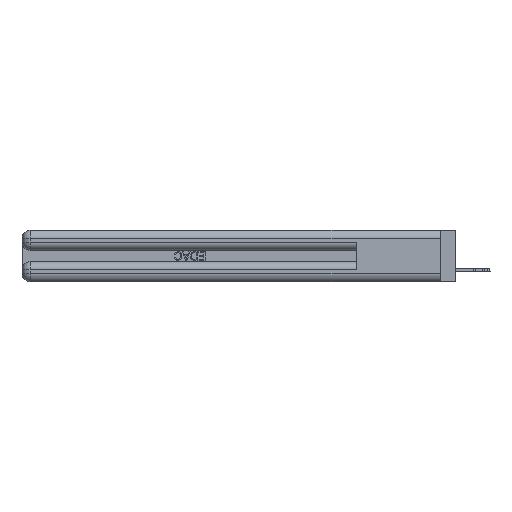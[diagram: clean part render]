
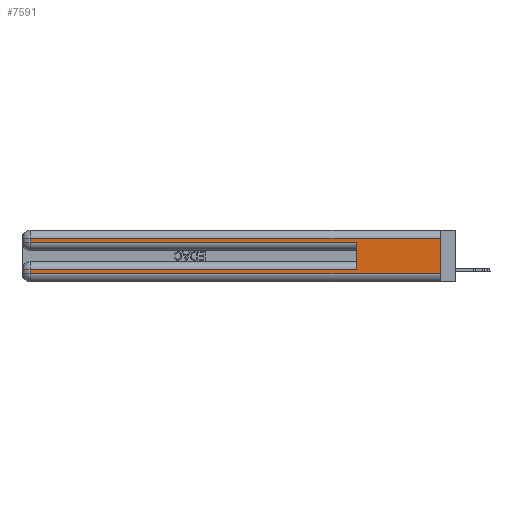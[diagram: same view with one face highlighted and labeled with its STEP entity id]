
A CAD part, left-side view. The second image highlights one B-rep face of the part: STEP entity #7591.
In plain terms, the highlighted planar face has unit normal (-1, 0, 0).
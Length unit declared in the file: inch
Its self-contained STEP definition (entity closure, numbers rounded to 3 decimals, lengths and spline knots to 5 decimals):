
#1581 = VECTOR ( 'NONE', #41209, 39.37008 ) ;
#2367 = LINE ( 'NONE', #12091, #41838 ) ;
#2590 = DIRECTION ( 'NONE',  ( 0., 0., 1. ) ) ;
#2711 = DIRECTION ( 'NONE',  ( 0., 0., -1. ) ) ;
#3112 = CARTESIAN_POINT ( 'NONE',  ( 0., 2.94, 0.06 ) ) ;
#5123 = EDGE_CURVE ( 'NONE', #44165, #44520, #13853, .T. ) ;
#5476 = VECTOR ( 'NONE', #2590, 39.37008 ) ;
#5653 = CARTESIAN_POINT ( 'NONE',  ( 0., 2.94, 0.285 ) ) ;
#5681 = LINE ( 'NONE', #5818, #33248 ) ;
#5818 = CARTESIAN_POINT ( 'NONE',  ( 0., 2.94, 0.37 ) ) ;
#6056 = CARTESIAN_POINT ( 'NONE',  ( 0., 2.94, 0.085 ) ) ;
#6322 = CARTESIAN_POINT ( 'NONE',  ( 0., 0., 0.085 ) ) ;
#6497 = EDGE_CURVE ( 'NONE', #46476, #43910, #26676, .T. ) ;
#6765 = DIRECTION ( 'NONE',  ( 1., 0., 0. ) ) ;
#7591 = ADVANCED_FACE ( 'NONE', ( #29410 ), #17162, .F. ) ;
#8442 = ORIENTED_EDGE ( 'NONE', *, *, #15375, .T. ) ;
#8867 = ORIENTED_EDGE ( 'NONE', *, *, #36440, .F. ) ;
#8888 = CARTESIAN_POINT ( 'NONE',  ( 0., 0.6, 0.285 ) ) ;
#9167 = VERTEX_POINT ( 'NONE', #3112 ) ;
#11822 = VERTEX_POINT ( 'NONE', #6056 ) ;
#11968 = LINE ( 'NONE', #39969, #27791 ) ;
#12091 = CARTESIAN_POINT ( 'NONE',  ( 0., 0., 0.285 ) ) ;
#13853 = LINE ( 'NONE', #43042, #22869 ) ;
#14096 = EDGE_CURVE ( 'NONE', #44520, #40627, #2367, .T. ) ;
#15375 = EDGE_CURVE ( 'NONE', #38462, #11822, #41088, .T. ) ;
#15749 = EDGE_LOOP ( 'NONE', ( #31934, #30500, #41858, #25301, #8867, #8442, #25909, #17855 ) ) ;
#16567 = CARTESIAN_POINT ( 'NONE',  ( 0., 0.6, 0.145 ) ) ;
#17162 = PLANE ( 'NONE',  #46320 ) ;
#17855 = ORIENTED_EDGE ( 'NONE', *, *, #39110, .T. ) ;
#18387 = DIRECTION ( 'NONE',  ( 0., -1., 0. ) ) ;
#19266 = CARTESIAN_POINT ( 'NONE',  ( 0., 0., 0.06 ) ) ;
#21285 = CARTESIAN_POINT ( 'NONE',  ( 0., 2.94, 0.31 ) ) ;
#21332 = DIRECTION ( 'NONE',  ( 0., 0., -1. ) ) ;
#21944 = EDGE_CURVE ( 'NONE', #46476, #44165, #25251, .T. ) ;
#22869 = VECTOR ( 'NONE', #36681, 39.37008 ) ;
#22954 = DIRECTION ( 'NONE',  ( 0., -1., 0. ) ) ;
#24744 = CARTESIAN_POINT ( 'NONE',  ( 0., 0.6, 0.085 ) ) ;
#25251 = LINE ( 'NONE', #37405, #1581 ) ;
#25301 = ORIENTED_EDGE ( 'NONE', *, *, #14096, .T. ) ;
#25400 = CARTESIAN_POINT ( 'NONE',  ( 0., 0., 0.37 ) ) ;
#25909 = ORIENTED_EDGE ( 'NONE', *, *, #34215, .T. ) ;
#26676 = LINE ( 'NONE', #25400, #42534 ) ;
#27791 = VECTOR ( 'NONE', #18387, 39.37008 ) ;
#28248 = DIRECTION ( 'NONE',  ( 0., 1., 0. ) ) ;
#29410 = FACE_OUTER_BOUND ( 'NONE', #15749, .T. ) ;
#30500 = ORIENTED_EDGE ( 'NONE', *, *, #21944, .T. ) ;
#31934 = ORIENTED_EDGE ( 'NONE', *, *, #6497, .F. ) ;
#32084 = VECTOR ( 'NONE', #28248, 39.37008 ) ;
#32495 = CARTESIAN_POINT ( 'NONE',  ( 0., 0., 0.31 ) ) ;
#33248 = VECTOR ( 'NONE', #34205, 39.37008 ) ;
#34205 = DIRECTION ( 'NONE',  ( 0., 0., -1. ) ) ;
#34215 = EDGE_CURVE ( 'NONE', #11822, #9167, #5681, .T. ) ;
#35346 = LINE ( 'NONE', #16567, #5476 ) ;
#36440 = EDGE_CURVE ( 'NONE', #38462, #40627, #35346, .T. ) ;
#36681 = DIRECTION ( 'NONE',  ( 0., 0., -1. ) ) ;
#37405 = CARTESIAN_POINT ( 'NONE',  ( 0., 0., 0.31 ) ) ;
#38462 = VERTEX_POINT ( 'NONE', #24744 ) ;
#39110 = EDGE_CURVE ( 'NONE', #9167, #43910, #11968, .T. ) ;
#39969 = CARTESIAN_POINT ( 'NONE',  ( 0., 0., 0.06 ) ) ;
#40627 = VERTEX_POINT ( 'NONE', #8888 ) ;
#41088 = LINE ( 'NONE', #6322, #32084 ) ;
#41209 = DIRECTION ( 'NONE',  ( 0., 1., 0. ) ) ;
#41838 = VECTOR ( 'NONE', #22954, 39.37008 ) ;
#41858 = ORIENTED_EDGE ( 'NONE', *, *, #5123, .T. ) ;
#42534 = VECTOR ( 'NONE', #21332, 39.37008 ) ;
#42912 = CARTESIAN_POINT ( 'NONE',  ( 0., 0., 0.37 ) ) ;
#43042 = CARTESIAN_POINT ( 'NONE',  ( 0., 2.94, 0.37 ) ) ;
#43910 = VERTEX_POINT ( 'NONE', #19266 ) ;
#44165 = VERTEX_POINT ( 'NONE', #21285 ) ;
#44520 = VERTEX_POINT ( 'NONE', #5653 ) ;
#46320 = AXIS2_PLACEMENT_3D ( 'NONE', #42912, #6765, #2711 ) ;
#46476 = VERTEX_POINT ( 'NONE', #32495 ) ;
